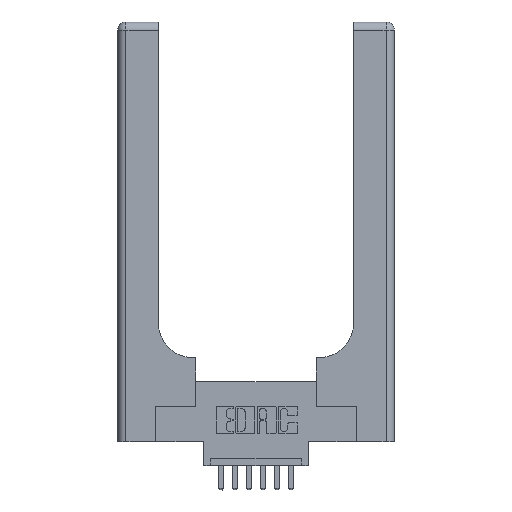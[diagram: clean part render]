
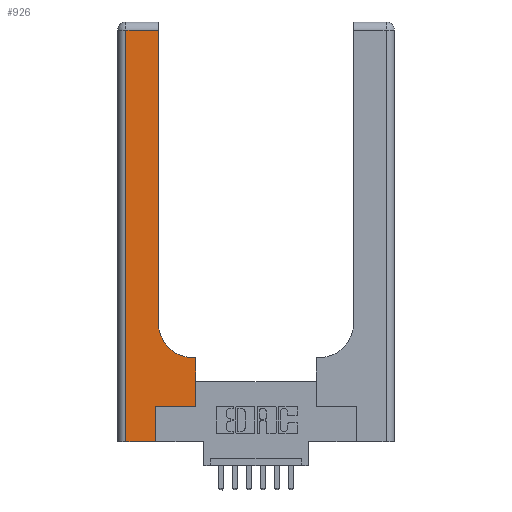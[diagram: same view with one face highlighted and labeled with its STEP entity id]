
A CAD part, top view. The second image highlights one B-rep face of the part: STEP entity #926.
In plain terms, the highlighted planar face has unit normal (0, 0, 1).
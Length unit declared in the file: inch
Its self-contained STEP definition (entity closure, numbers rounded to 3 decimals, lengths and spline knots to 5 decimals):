
#65 = DIRECTION ( 'NONE',  ( 1., 0., 0. ) ) ;
#108 = CARTESIAN_POINT ( 'NONE',  ( 0.2915, 3., 0.37 ) ) ;
#119 = CARTESIAN_POINT ( 'NONE',  ( 0., 0., 0.37 ) ) ;
#350 = CARTESIAN_POINT ( 'NONE',  ( 0.2915, 0.85, 0.37 ) ) ;
#642 = VERTEX_POINT ( 'NONE', #11237 ) ;
#675 = CARTESIAN_POINT ( 'NONE',  ( 0.269, 0.25, 0.37 ) ) ;
#684 = EDGE_CURVE ( 'NONE', #9678, #2153, #8254, .T. ) ;
#769 = LINE ( 'NONE', #3743, #5766 ) ;
#926 = ADVANCED_FACE ( 'NONE', ( #11156 ), #9748, .F. ) ;
#1099 = DIRECTION ( 'NONE',  ( -1., 0., 0. ) ) ;
#1173 = ORIENTED_EDGE ( 'NONE', *, *, #3280, .T. ) ;
#1236 = AXIS2_PLACEMENT_3D ( 'NONE', #13244, #2929, #12110 ) ;
#1311 = VECTOR ( 'NONE', #6756, 39.37008 ) ;
#1349 = DIRECTION ( 'NONE',  ( 0., 0., -1. ) ) ;
#2153 = VERTEX_POINT ( 'NONE', #9861 ) ;
#2280 = EDGE_LOOP ( 'NONE', ( #14305, #1173, #6563, #6585, #8145, #2968, #5141, #8135, #4266 ) ) ;
#2553 = LINE ( 'NONE', #5327, #8447 ) ;
#2746 = EDGE_CURVE ( 'NONE', #2153, #642, #2553, .T. ) ;
#2882 = LINE ( 'NONE', #119, #4137 ) ;
#2897 = EDGE_CURVE ( 'NONE', #642, #6507, #13837, .T. ) ;
#2929 = DIRECTION ( 'NONE',  ( 0., 0., -1. ) ) ;
#2968 = ORIENTED_EDGE ( 'NONE', *, *, #684, .T. ) ;
#3128 = EDGE_CURVE ( 'NONE', #10225, #11516, #769, .T. ) ;
#3260 = VECTOR ( 'NONE', #10203, 39.37008 ) ;
#3280 = EDGE_CURVE ( 'NONE', #14656, #10225, #9716, .T. ) ;
#3463 = EDGE_CURVE ( 'NONE', #11516, #7473, #2882, .T. ) ;
#3721 = DIRECTION ( 'NONE',  ( 0., 1., 0. ) ) ;
#3743 = CARTESIAN_POINT ( 'NONE',  ( 0.06, 3., 0.37 ) ) ;
#4041 = CARTESIAN_POINT ( 'NONE',  ( 0.2915, 2.94, 0.37 ) ) ;
#4137 = VECTOR ( 'NONE', #65, 39.37008 ) ;
#4266 = ORIENTED_EDGE ( 'NONE', *, *, #7236, .T. ) ;
#5141 = ORIENTED_EDGE ( 'NONE', *, *, #2746, .T. ) ;
#5238 = VERTEX_POINT ( 'NONE', #350 ) ;
#5275 = EDGE_CURVE ( 'NONE', #7473, #9678, #9857, .T. ) ;
#5327 = CARTESIAN_POINT ( 'NONE',  ( 0.5585, 0.25, 0.37 ) ) ;
#5725 = CARTESIAN_POINT ( 'NONE',  ( 0.2915, 0.6, 0.37 ) ) ;
#5766 = VECTOR ( 'NONE', #8303, 39.37008 ) ;
#6148 = CARTESIAN_POINT ( 'NONE',  ( 0.269, 0., 0.37 ) ) ;
#6365 = CARTESIAN_POINT ( 'NONE',  ( 0., 2.94, 0.37 ) ) ;
#6408 = DIRECTION ( 'NONE',  ( -1., 0., 0. ) ) ;
#6426 = DIRECTION ( 'NONE',  ( 0., 1., 0. ) ) ;
#6507 = VERTEX_POINT ( 'NONE', #7009 ) ;
#6563 = ORIENTED_EDGE ( 'NONE', *, *, #3128, .T. ) ;
#6585 = ORIENTED_EDGE ( 'NONE', *, *, #3463, .T. ) ;
#6756 = DIRECTION ( 'NONE',  ( 0., 1., 0. ) ) ;
#7009 = CARTESIAN_POINT ( 'NONE',  ( 0.5415, 0.6, 0.37 ) ) ;
#7095 = CIRCLE ( 'NONE', #8074, 0.25 ) ;
#7236 = EDGE_CURVE ( 'NONE', #6507, #5238, #7095, .T. ) ;
#7473 = VERTEX_POINT ( 'NONE', #8319 ) ;
#8074 = AXIS2_PLACEMENT_3D ( 'NONE', #10462, #1349, #13849 ) ;
#8135 = ORIENTED_EDGE ( 'NONE', *, *, #2897, .T. ) ;
#8145 = ORIENTED_EDGE ( 'NONE', *, *, #5275, .T. ) ;
#8254 = LINE ( 'NONE', #675, #3260 ) ;
#8303 = DIRECTION ( 'NONE',  ( 0., -1., 0. ) ) ;
#8319 = CARTESIAN_POINT ( 'NONE',  ( 0.269, 0., 0.37 ) ) ;
#8447 = VECTOR ( 'NONE', #6426, 39.37008 ) ;
#8536 = CARTESIAN_POINT ( 'NONE',  ( 0.269, 0.25, 0.37 ) ) ;
#9678 = VERTEX_POINT ( 'NONE', #8536 ) ;
#9715 = LINE ( 'NONE', #108, #1311 ) ;
#9716 = LINE ( 'NONE', #6365, #14712 ) ;
#9748 = PLANE ( 'NONE',  #1236 ) ;
#9857 = LINE ( 'NONE', #6148, #10586 ) ;
#9861 = CARTESIAN_POINT ( 'NONE',  ( 0.5585, 0.25, 0.37 ) ) ;
#9975 = CARTESIAN_POINT ( 'NONE',  ( 0.06, 0., 0.37 ) ) ;
#10203 = DIRECTION ( 'NONE',  ( 1., 0., 0. ) ) ;
#10225 = VERTEX_POINT ( 'NONE', #11807 ) ;
#10462 = CARTESIAN_POINT ( 'NONE',  ( 0.5415, 0.85, 0.37 ) ) ;
#10586 = VECTOR ( 'NONE', #3721, 39.37008 ) ;
#10807 = VECTOR ( 'NONE', #1099, 39.37008 ) ;
#11156 = FACE_OUTER_BOUND ( 'NONE', #2280, .T. ) ;
#11237 = CARTESIAN_POINT ( 'NONE',  ( 0.5585, 0.6, 0.37 ) ) ;
#11516 = VERTEX_POINT ( 'NONE', #9975 ) ;
#11560 = EDGE_CURVE ( 'NONE', #5238, #14656, #9715, .T. ) ;
#11807 = CARTESIAN_POINT ( 'NONE',  ( 0.06, 2.94, 0.37 ) ) ;
#12110 = DIRECTION ( 'NONE',  ( -1., 0., 0. ) ) ;
#13244 = CARTESIAN_POINT ( 'NONE',  ( 0., 3., 0.37 ) ) ;
#13837 = LINE ( 'NONE', #5725, #10807 ) ;
#13849 = DIRECTION ( 'NONE',  ( 1., 0., 0. ) ) ;
#14305 = ORIENTED_EDGE ( 'NONE', *, *, #11560, .T. ) ;
#14656 = VERTEX_POINT ( 'NONE', #4041 ) ;
#14712 = VECTOR ( 'NONE', #6408, 39.37008 ) ;
